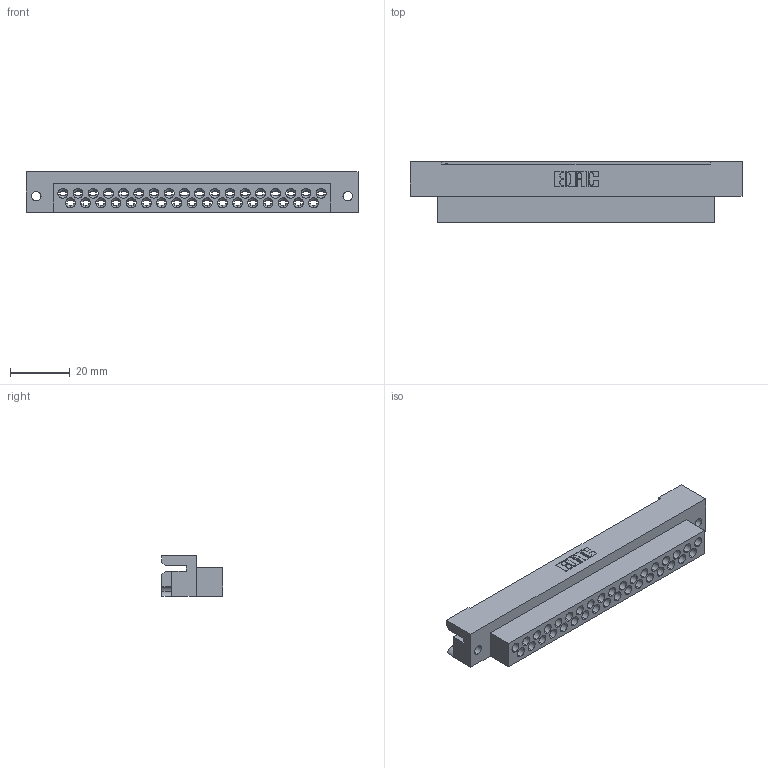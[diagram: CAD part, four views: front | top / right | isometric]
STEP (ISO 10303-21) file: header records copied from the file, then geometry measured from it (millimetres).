
FILE_DESCRIPTION (( 'STEP AP203' ), '1' );
FILE_NAME ('438-035-000-122.STEP', '2020-03-12T20:46:23', ( '' ), ( '' ), 'SwSTEP 2.0', 'SolidWorks 2016', '' );
FILE_SCHEMA (( 'CONFIG_CONTROL_DESIGN' ));
Length unit declared in the file: millimetre
Products named in the file (2): 438-035-000-122; 438-210-001_438-210-035-112
Assembly tree (1 placements, depth 2):
  438-035-000-122
    438-210-001_438-210-035-112
Bounding box: 111 x 20.45 x 13.49 mm (x, y, z)
Volume: 16941.3 mm3; surface area: 16777.4 mm2
Topology: 1 solids, 1 shells, 1066 faces, 3166 edges, 2075 vertices
Faces by surface type: plane 819, cylinder 120, cone 105, bspline 22
Entity records: 36977 total; most frequent: CARTESIAN_POINT 8657, ORIENTED_EDGE 6332, DIRECTION 5285, EDGE_CURVE 3166, LINE 2215, VECTOR 2215, VERTEX_POINT 2075, AXIS2_PLACEMENT_3D 1535
